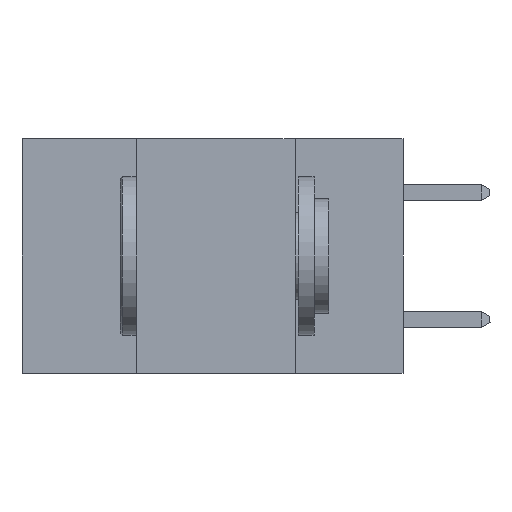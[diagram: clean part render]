
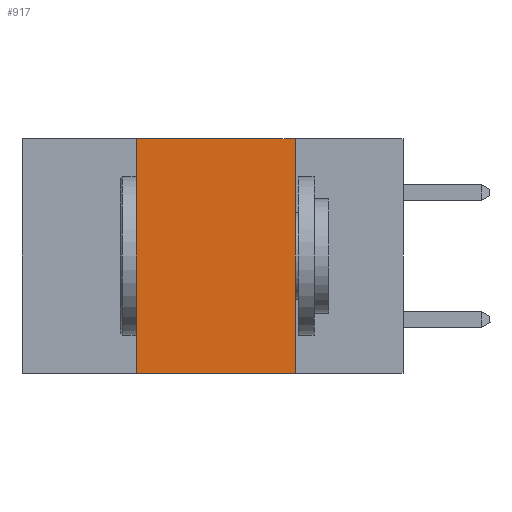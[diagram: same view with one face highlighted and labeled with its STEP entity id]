
A CAD part, left-side view. The second image highlights one B-rep face of the part: STEP entity #917.
In plain terms, the highlighted planar face has unit normal (-1, 0, 0).
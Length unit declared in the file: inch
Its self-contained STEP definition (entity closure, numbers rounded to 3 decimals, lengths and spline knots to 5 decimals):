
#351 = ORIENTED_EDGE ( 'NONE', *, *, #9944, .F. ) ;
#549 = CARTESIAN_POINT ( 'NONE',  ( 0., 0.42, -0.37 ) ) ;
#694 = CARTESIAN_POINT ( 'NONE',  ( 0., 0.6, -0.37 ) ) ;
#735 = VERTEX_POINT ( 'NONE', #11770 ) ;
#917 = ADVANCED_FACE ( 'NONE', ( #8062 ), #15263, .F. ) ;
#1036 = VECTOR ( 'NONE', #5411, 39.37008 ) ;
#1656 = EDGE_CURVE ( 'NONE', #17901, #735, #24271, .T. ) ;
#2127 = EDGE_CURVE ( 'NONE', #7574, #13693, #9581, .T. ) ;
#3012 = DIRECTION ( 'NONE',  ( 0., -1., 0. ) ) ;
#4563 = CARTESIAN_POINT ( 'NONE',  ( 0., 0.42, 0. ) ) ;
#4867 = ORIENTED_EDGE ( 'NONE', *, *, #19074, .F. ) ;
#5411 = DIRECTION ( 'NONE',  ( 0., -1., 0. ) ) ;
#5901 = DIRECTION ( 'NONE',  ( 0., 0., -1. ) ) ;
#6071 = VECTOR ( 'NONE', #12257, 39.37008 ) ;
#7134 = DIRECTION ( 'NONE',  ( 0., 0., 1. ) ) ;
#7368 = VECTOR ( 'NONE', #3012, 39.37008 ) ;
#7574 = VERTEX_POINT ( 'NONE', #4563 ) ;
#8062 = FACE_OUTER_BOUND ( 'NONE', #15213, .T. ) ;
#9581 = LINE ( 'NONE', #24025, #7368 ) ;
#9944 = EDGE_CURVE ( 'NONE', #17901, #7574, #13047, .T. ) ;
#11640 = ORIENTED_EDGE ( 'NONE', *, *, #2127, .F. ) ;
#11770 = CARTESIAN_POINT ( 'NONE',  ( 0., 0.17, -0.37 ) ) ;
#12257 = DIRECTION ( 'NONE',  ( 0., 0., -1. ) ) ;
#13047 = LINE ( 'NONE', #30129, #13810 ) ;
#13693 = VERTEX_POINT ( 'NONE', #14073 ) ;
#13810 = VECTOR ( 'NONE', #7134, 39.37008 ) ;
#14073 = CARTESIAN_POINT ( 'NONE',  ( 0., 0.17, 0. ) ) ;
#15213 = EDGE_LOOP ( 'NONE', ( #4867, #11640, #351, #29029 ) ) ;
#15263 = PLANE ( 'NONE',  #18734 ) ;
#17901 = VERTEX_POINT ( 'NONE', #549 ) ;
#18209 = LINE ( 'NONE', #26401, #6071 ) ;
#18734 = AXIS2_PLACEMENT_3D ( 'NONE', #24885, #29321, #5901 ) ;
#19074 = EDGE_CURVE ( 'NONE', #13693, #735, #18209, .T. ) ;
#24025 = CARTESIAN_POINT ( 'NONE',  ( 0., 0.6, 0. ) ) ;
#24271 = LINE ( 'NONE', #694, #1036 ) ;
#24885 = CARTESIAN_POINT ( 'NONE',  ( 0., 0.6, 0. ) ) ;
#26401 = CARTESIAN_POINT ( 'NONE',  ( 0., 0.17, 0. ) ) ;
#29029 = ORIENTED_EDGE ( 'NONE', *, *, #1656, .T. ) ;
#29321 = DIRECTION ( 'NONE',  ( 1., 0., 0. ) ) ;
#30129 = CARTESIAN_POINT ( 'NONE',  ( 0., 0.42, 0. ) ) ;
